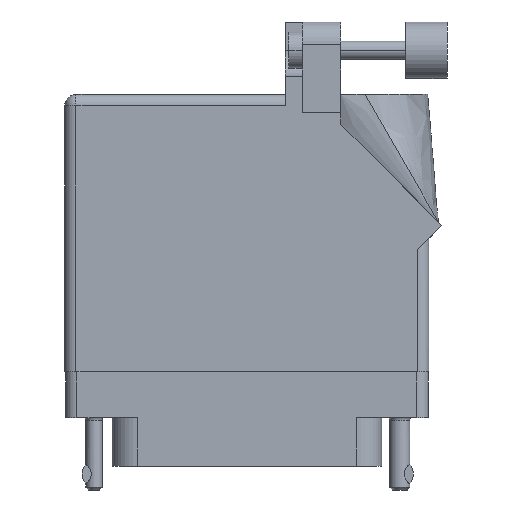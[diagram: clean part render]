
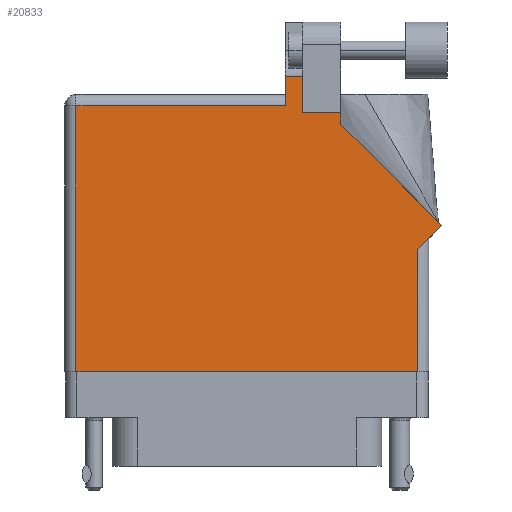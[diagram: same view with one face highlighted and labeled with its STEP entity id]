
A CAD part, front view. The second image highlights one B-rep face of the part: STEP entity #20833.
In plain terms, the highlighted face is planar.
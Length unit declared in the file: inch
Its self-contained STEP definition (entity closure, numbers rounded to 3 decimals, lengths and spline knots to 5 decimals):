
#442 = EDGE_CURVE ( 'NONE', #23372, #46192, #4627, .T. ) ;
#462 = VERTEX_POINT ( 'NONE', #31204 ) ;
#605 = CARTESIAN_POINT ( 'NONE',  ( 1.07571, 0.70771, 0.455 ) ) ;
#1259 = VECTOR ( 'NONE', #29245, 39.37008 ) ;
#3327 = ORIENTED_EDGE ( 'NONE', *, *, #14382, .T. ) ;
#4584 = CARTESIAN_POINT ( 'NONE',  ( 0.519, 1.33, 0.455 ) ) ;
#4627 = LINE ( 'NONE', #24664, #26136 ) ;
#5095 = DIRECTION ( 'NONE',  ( 0., -1., 0. ) ) ;
#5291 = DIRECTION ( 'NONE',  ( -1., 0., 0. ) ) ;
#5724 = LINE ( 'NONE', #45528, #47666 ) ;
#6283 = VECTOR ( 'NONE', #42641, 39.37008 ) ;
#6970 = ORIENTED_EDGE ( 'NONE', *, *, #34557, .T. ) ;
#7189 = DIRECTION ( 'NONE',  ( 0.707, 0.707, 0. ) ) ;
#7644 = CARTESIAN_POINT ( 'NONE',  ( 1.07571, 0.70771, 0.455 ) ) ;
#8861 = LINE ( 'NONE', #605, #13017 ) ;
#9146 = LINE ( 'NONE', #29588, #19295 ) ;
#10541 = DIRECTION ( 'NONE',  ( -1., 0., 0. ) ) ;
#11073 = ORIENTED_EDGE ( 'NONE', *, *, #33075, .T. ) ;
#13017 = VECTOR ( 'NONE', #27143, 39.37008 ) ;
#13764 = EDGE_CURVE ( 'NONE', #22980, #23372, #23541, .T. ) ;
#13780 = LINE ( 'NONE', #44197, #1259 ) ;
#14327 = CARTESIAN_POINT ( 'NONE',  ( 0.306, 1.33, 0.455 ) ) ;
#14382 = EDGE_CURVE ( 'NONE', #27236, #33471, #9146, .T. ) ;
#14588 = DIRECTION ( 'NONE',  ( -1., 0., 0. ) ) ;
#15031 = VERTEX_POINT ( 'NONE', #45329 ) ;
#15198 = EDGE_CURVE ( 'NONE', #15329, #27236, #34191, .T. ) ;
#15329 = VERTEX_POINT ( 'NONE', #25105 ) ;
#16759 = LINE ( 'NONE', #17310, #28137 ) ;
#17310 = CARTESIAN_POINT ( 'NONE',  ( 0.63677, 1.5315, 0.455 ) ) ;
#19295 = VECTOR ( 'NONE', #10541, 39.37008 ) ;
#20364 = VERTEX_POINT ( 'NONE', #48502 ) ;
#20806 = PLANE ( 'NONE',  #45549 ) ;
#20833 = ADVANCED_FACE ( 'NONE', ( #27093 ), #20806, .F. ) ;
#21256 = LINE ( 'NONE', #42986, #6283 ) ;
#21308 = CARTESIAN_POINT ( 'NONE',  ( 0.519, 1.26442, 0.455 ) ) ;
#22216 = CARTESIAN_POINT ( 'NONE',  ( -0.943, 1.368, 0.455 ) ) ;
#22826 = EDGE_LOOP ( 'NONE', ( #45573, #6970, #34079, #3327, #47589, #11073, #35393, #27155, #30211, #38154, #42798 ) ) ;
#22980 = VERTEX_POINT ( 'NONE', #4584 ) ;
#23265 = VECTOR ( 'NONE', #32883, 39.37008 ) ;
#23372 = VERTEX_POINT ( 'NONE', #14327 ) ;
#23541 = LINE ( 'NONE', #33500, #43354 ) ;
#24453 = CARTESIAN_POINT ( 'NONE',  ( 0.212, 1.43, 0.455 ) ) ;
#24664 = CARTESIAN_POINT ( 'NONE',  ( 0.306, 1.33, 0.455 ) ) ;
#25105 = CARTESIAN_POINT ( 'NONE',  ( 0.212, 1.5315, 0.455 ) ) ;
#26136 = VECTOR ( 'NONE', #35904, 39.37008 ) ;
#26619 = EDGE_CURVE ( 'NONE', #38037, #20364, #47839, .T. ) ;
#26927 = EDGE_CURVE ( 'NONE', #47030, #15031, #8861, .T. ) ;
#27093 = FACE_OUTER_BOUND ( 'NONE', #22826, .T. ) ;
#27143 = DIRECTION ( 'NONE',  ( -0.707, 0.707, 0. ) ) ;
#27155 = ORIENTED_EDGE ( 'NONE', *, *, #44939, .T. ) ;
#27236 = VERTEX_POINT ( 'NONE', #47616 ) ;
#28137 = VECTOR ( 'NONE', #36237, 39.37008 ) ;
#28984 = CARTESIAN_POINT ( 'NONE',  ( 0.943, -0.1, 0.455 ) ) ;
#29005 = CARTESIAN_POINT ( 'NONE',  ( 0.943, 0.637, 0.455 ) ) ;
#29102 = LINE ( 'NONE', #21308, #47713 ) ;
#29245 = DIRECTION ( 'NONE',  ( 1., 0., 0. ) ) ;
#29588 = CARTESIAN_POINT ( 'NONE',  ( -1.005, 1.368, 0.455 ) ) ;
#30211 = ORIENTED_EDGE ( 'NONE', *, *, #26927, .T. ) ;
#31204 = CARTESIAN_POINT ( 'NONE',  ( -0.943, -0.1, 0.455 ) ) ;
#32676 = DIRECTION ( 'NONE',  ( 0., 1., 0. ) ) ;
#32883 = DIRECTION ( 'NONE',  ( 0., 1., 0. ) ) ;
#33075 = EDGE_CURVE ( 'NONE', #462, #38037, #13780, .T. ) ;
#33471 = VERTEX_POINT ( 'NONE', #22216 ) ;
#33500 = CARTESIAN_POINT ( 'NONE',  ( 0.519, 1.33, 0.455 ) ) ;
#34079 = ORIENTED_EDGE ( 'NONE', *, *, #15198, .T. ) ;
#34191 = LINE ( 'NONE', #24453, #42626 ) ;
#34557 = EDGE_CURVE ( 'NONE', #46192, #15329, #16759, .T. ) ;
#35393 = ORIENTED_EDGE ( 'NONE', *, *, #26619, .T. ) ;
#35541 = CARTESIAN_POINT ( 'NONE',  ( -1.005, 1.43, 0.455 ) ) ;
#35904 = DIRECTION ( 'NONE',  ( 0., 1., 0. ) ) ;
#36237 = DIRECTION ( 'NONE',  ( -1., 0., 0. ) ) ;
#38037 = VERTEX_POINT ( 'NONE', #28984 ) ;
#38154 = ORIENTED_EDGE ( 'NONE', *, *, #44243, .T. ) ;
#42626 = VECTOR ( 'NONE', #5095, 39.37008 ) ;
#42641 = DIRECTION ( 'NONE',  ( 0., -1., 0. ) ) ;
#42798 = ORIENTED_EDGE ( 'NONE', *, *, #13764, .T. ) ;
#42986 = CARTESIAN_POINT ( 'NONE',  ( -0.943, -0.1, 0.455 ) ) ;
#43354 = VECTOR ( 'NONE', #14588, 39.37008 ) ;
#44197 = CARTESIAN_POINT ( 'NONE',  ( -1.005, -0.1, 0.455 ) ) ;
#44243 = EDGE_CURVE ( 'NONE', #15031, #22980, #29102, .T. ) ;
#44939 = EDGE_CURVE ( 'NONE', #20364, #47030, #5724, .T. ) ;
#45057 = EDGE_CURVE ( 'NONE', #33471, #462, #21256, .T. ) ;
#45329 = CARTESIAN_POINT ( 'NONE',  ( 0.519, 1.26442, 0.455 ) ) ;
#45528 = CARTESIAN_POINT ( 'NONE',  ( 1.005, 0.637, 0.455 ) ) ;
#45549 = AXIS2_PLACEMENT_3D ( 'NONE', #35541, #47130, #5291 ) ;
#45573 = ORIENTED_EDGE ( 'NONE', *, *, #442, .T. ) ;
#46192 = VERTEX_POINT ( 'NONE', #48087 ) ;
#47030 = VERTEX_POINT ( 'NONE', #7644 ) ;
#47130 = DIRECTION ( 'NONE',  ( 0., 0., -1. ) ) ;
#47589 = ORIENTED_EDGE ( 'NONE', *, *, #45057, .T. ) ;
#47616 = CARTESIAN_POINT ( 'NONE',  ( 0.212, 1.368, 0.455 ) ) ;
#47666 = VECTOR ( 'NONE', #7189, 39.37008 ) ;
#47713 = VECTOR ( 'NONE', #32676, 39.37008 ) ;
#47839 = LINE ( 'NONE', #29005, #23265 ) ;
#48087 = CARTESIAN_POINT ( 'NONE',  ( 0.306, 1.5315, 0.455 ) ) ;
#48502 = CARTESIAN_POINT ( 'NONE',  ( 0.943, 0.575, 0.455 ) ) ;
